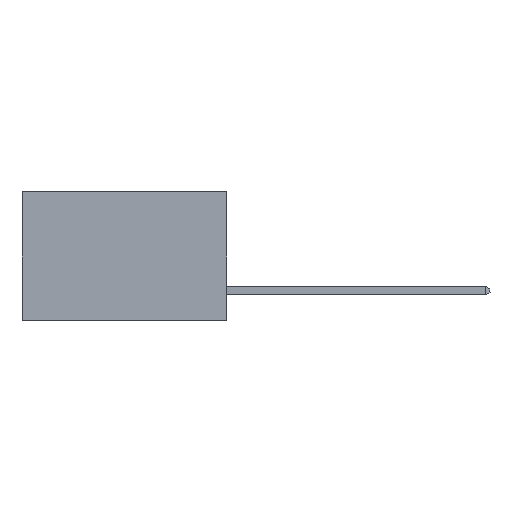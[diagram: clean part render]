
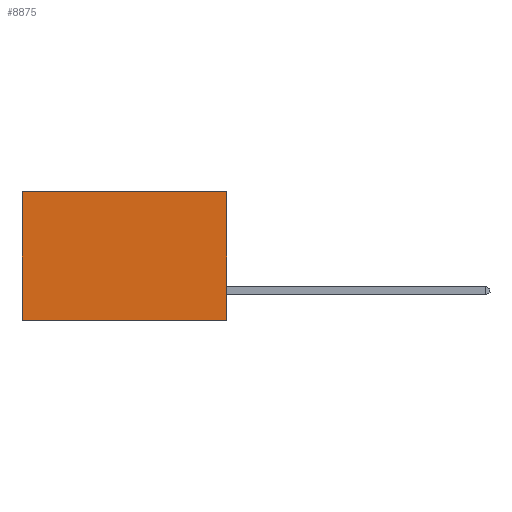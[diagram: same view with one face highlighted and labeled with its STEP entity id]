
A CAD part, left-side view. The second image highlights one B-rep face of the part: STEP entity #8875.
In plain terms, the highlighted planar face has unit normal (-1, 0, 0).
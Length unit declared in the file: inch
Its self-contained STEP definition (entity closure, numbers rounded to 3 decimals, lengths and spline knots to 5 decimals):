
#56 = EDGE_CURVE ( 'NONE', #6586, #2580, #1073, .T. ) ;
#577 = CARTESIAN_POINT ( 'NONE',  ( 0.277, 0., -0.37 ) ) ;
#667 = ORIENTED_EDGE ( 'NONE', *, *, #7822, .F. ) ;
#688 = ORIENTED_EDGE ( 'NONE', *, *, #1442, .F. ) ;
#721 = ORIENTED_EDGE ( 'NONE', *, *, #56, .T. ) ;
#1073 = LINE ( 'NONE', #4070, #8825 ) ;
#1275 = EDGE_LOOP ( 'NONE', ( #4801, #667, #688, #721 ) ) ;
#1442 = EDGE_CURVE ( 'NONE', #6586, #3844, #3156, .T. ) ;
#1811 = VECTOR ( 'NONE', #3408, 39.37008 ) ;
#2160 = AXIS2_PLACEMENT_3D ( 'NONE', #4685, #4656, #4584 ) ;
#2171 = EDGE_CURVE ( 'NONE', #2580, #4679, #8898, .T. ) ;
#2212 = CARTESIAN_POINT ( 'NONE',  ( 0.277, 0.59, 0. ) ) ;
#2283 = CARTESIAN_POINT ( 'NONE',  ( 0.277, 0., 0. ) ) ;
#2580 = VERTEX_POINT ( 'NONE', #2212 ) ;
#2735 = DIRECTION ( 'NONE',  ( 0., 0., -1. ) ) ;
#3156 = LINE ( 'NONE', #577, #8799 ) ;
#3249 = CARTESIAN_POINT ( 'NONE',  ( 0.277, 0.59, -0.37 ) ) ;
#3324 = CARTESIAN_POINT ( 'NONE',  ( 0.277, 0., -0.37 ) ) ;
#3363 = CARTESIAN_POINT ( 'NONE',  ( 0.277, 0., -0.37 ) ) ;
#3408 = DIRECTION ( 'NONE',  ( 0., 1., 0. ) ) ;
#3844 = VERTEX_POINT ( 'NONE', #3363 ) ;
#4070 = CARTESIAN_POINT ( 'NONE',  ( 0.277, 0., 0. ) ) ;
#4331 = DIRECTION ( 'NONE',  ( 0., 1., 0. ) ) ;
#4483 = DIRECTION ( 'NONE',  ( 0., 0., -1. ) ) ;
#4584 = DIRECTION ( 'NONE',  ( 0., 0., -1. ) ) ;
#4656 = DIRECTION ( 'NONE',  ( 1., 0., 0. ) ) ;
#4679 = VERTEX_POINT ( 'NONE', #3249 ) ;
#4685 = CARTESIAN_POINT ( 'NONE',  ( 0.277, 0., -0.37 ) ) ;
#4759 = FACE_OUTER_BOUND ( 'NONE', #1275, .T. ) ;
#4801 = ORIENTED_EDGE ( 'NONE', *, *, #2171, .T. ) ;
#4849 = PLANE ( 'NONE',  #2160 ) ;
#6586 = VERTEX_POINT ( 'NONE', #2283 ) ;
#7011 = VECTOR ( 'NONE', #2735, 39.37008 ) ;
#7822 = EDGE_CURVE ( 'NONE', #3844, #4679, #8031, .T. ) ;
#8031 = LINE ( 'NONE', #3324, #1811 ) ;
#8389 = CARTESIAN_POINT ( 'NONE',  ( 0.277, 0.59, -0.37 ) ) ;
#8799 = VECTOR ( 'NONE', #4483, 39.37008 ) ;
#8825 = VECTOR ( 'NONE', #4331, 39.37008 ) ;
#8875 = ADVANCED_FACE ( 'NONE', ( #4759 ), #4849, .F. ) ;
#8898 = LINE ( 'NONE', #8389, #7011 ) ;
